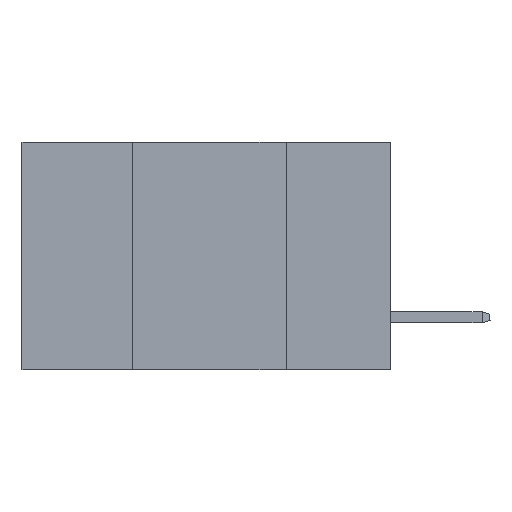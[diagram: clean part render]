
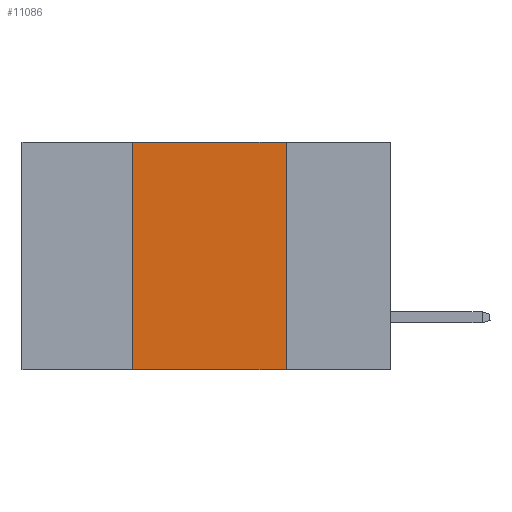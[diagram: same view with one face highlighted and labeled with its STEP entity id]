
A CAD part, left-side view. The second image highlights one B-rep face of the part: STEP entity #11086.
In plain terms, the highlighted planar face has unit normal (-1, 0, 0).
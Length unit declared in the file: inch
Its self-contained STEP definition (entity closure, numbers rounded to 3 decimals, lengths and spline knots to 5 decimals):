
#403 = CARTESIAN_POINT ( 'NONE',  ( 0., 0.42, 0. ) ) ;
#776 = VECTOR ( 'NONE', #6423, 39.37008 ) ;
#1090 = ORIENTED_EDGE ( 'NONE', *, *, #7427, .F. ) ;
#1524 = LINE ( 'NONE', #2025, #776 ) ;
#1562 = DIRECTION ( 'NONE',  ( 0., 0., -1. ) ) ;
#1669 = CARTESIAN_POINT ( 'NONE',  ( 0., 0.17, 0. ) ) ;
#1722 = EDGE_CURVE ( 'NONE', #4923, #2457, #10832, .T. ) ;
#2025 = CARTESIAN_POINT ( 'NONE',  ( 0., 0.6, 0. ) ) ;
#2321 = VECTOR ( 'NONE', #3642, 39.37008 ) ;
#2457 = VERTEX_POINT ( 'NONE', #12395 ) ;
#3642 = DIRECTION ( 'NONE',  ( 0., -1., 0. ) ) ;
#4739 = ORIENTED_EDGE ( 'NONE', *, *, #11955, .F. ) ;
#4781 = VERTEX_POINT ( 'NONE', #403 ) ;
#4923 = VERTEX_POINT ( 'NONE', #13326 ) ;
#5569 = DIRECTION ( 'NONE',  ( 0., 0., -1. ) ) ;
#5868 = CARTESIAN_POINT ( 'NONE',  ( 0., 0.6, -0.37 ) ) ;
#6215 = LINE ( 'NONE', #7927, #13969 ) ;
#6423 = DIRECTION ( 'NONE',  ( 0., -1., 0. ) ) ;
#6636 = PLANE ( 'NONE',  #9228 ) ;
#6658 = CARTESIAN_POINT ( 'NONE',  ( 0., 0.17, 0. ) ) ;
#6817 = LINE ( 'NONE', #1669, #7904 ) ;
#6834 = ORIENTED_EDGE ( 'NONE', *, *, #1722, .T. ) ;
#6957 = EDGE_LOOP ( 'NONE', ( #4739, #7525, #1090, #6834 ) ) ;
#7427 = EDGE_CURVE ( 'NONE', #4923, #4781, #6215, .T. ) ;
#7525 = ORIENTED_EDGE ( 'NONE', *, *, #13316, .F. ) ;
#7904 = VECTOR ( 'NONE', #1562, 39.37008 ) ;
#7927 = CARTESIAN_POINT ( 'NONE',  ( 0., 0.42, 0. ) ) ;
#8984 = VERTEX_POINT ( 'NONE', #6658 ) ;
#9013 = DIRECTION ( 'NONE',  ( 0., 0., 1. ) ) ;
#9228 = AXIS2_PLACEMENT_3D ( 'NONE', #11079, #9886, #5569 ) ;
#9831 = FACE_OUTER_BOUND ( 'NONE', #6957, .T. ) ;
#9886 = DIRECTION ( 'NONE',  ( 1., 0., 0. ) ) ;
#10832 = LINE ( 'NONE', #5868, #2321 ) ;
#11079 = CARTESIAN_POINT ( 'NONE',  ( 0., 0.6, 0. ) ) ;
#11086 = ADVANCED_FACE ( 'NONE', ( #9831 ), #6636, .F. ) ;
#11955 = EDGE_CURVE ( 'NONE', #8984, #2457, #6817, .T. ) ;
#12395 = CARTESIAN_POINT ( 'NONE',  ( 0., 0.17, -0.37 ) ) ;
#13316 = EDGE_CURVE ( 'NONE', #4781, #8984, #1524, .T. ) ;
#13326 = CARTESIAN_POINT ( 'NONE',  ( 0., 0.42, -0.37 ) ) ;
#13969 = VECTOR ( 'NONE', #9013, 39.37008 ) ;
